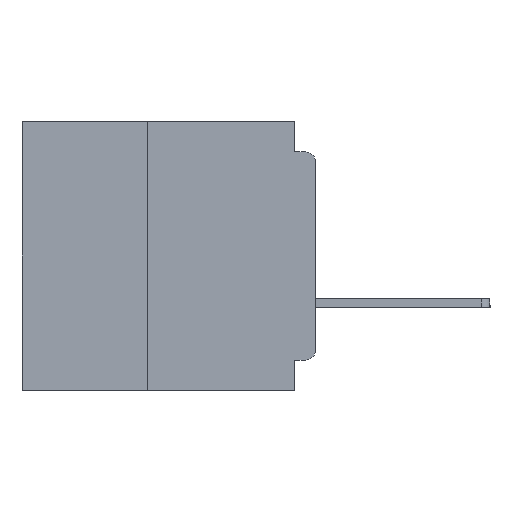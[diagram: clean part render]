
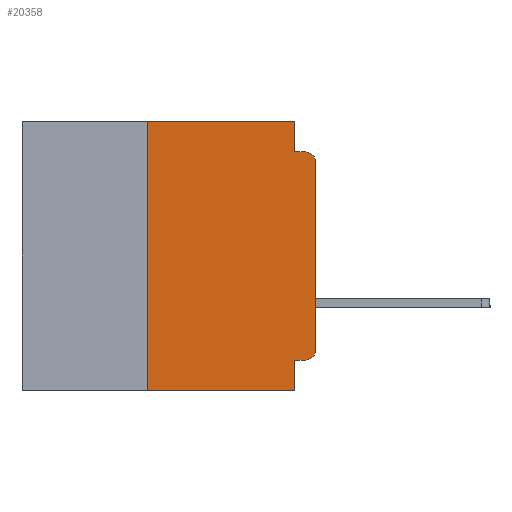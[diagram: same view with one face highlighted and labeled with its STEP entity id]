
A CAD part, left-side view. The second image highlights one B-rep face of the part: STEP entity #20358.
In plain terms, the highlighted planar face has unit normal (-1, 0, 0).
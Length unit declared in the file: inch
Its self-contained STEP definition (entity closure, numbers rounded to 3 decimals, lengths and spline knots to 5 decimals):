
#135 = EDGE_CURVE ( 'NONE', #14110, #29650, #40078, .T. ) ;
#1455 = CARTESIAN_POINT ( 'NONE',  ( 0., 0.437, -0.4 ) ) ;
#1759 = VECTOR ( 'NONE', #25606, 39.37008 ) ;
#2376 = CARTESIAN_POINT ( 'NONE',  ( 0., 0., -0.06 ) ) ;
#2440 = VERTEX_POINT ( 'NONE', #45266 ) ;
#2947 = VECTOR ( 'NONE', #39815, 39.37008 ) ;
#3290 = CARTESIAN_POINT ( 'NONE',  ( 0., 0., -0.34 ) ) ;
#3798 = ORIENTED_EDGE ( 'NONE', *, *, #34696, .F. ) ;
#3933 = VERTEX_POINT ( 'NONE', #2376 ) ;
#4945 = DIRECTION ( 'NONE',  ( 1., 0., 0. ) ) ;
#4977 = DIRECTION ( 'NONE',  ( 0., 0., 1. ) ) ;
#5087 = CARTESIAN_POINT ( 'NONE',  ( 0., 0.031, -0.4 ) ) ;
#6146 = LINE ( 'NONE', #5087, #36688 ) ;
#6580 = FACE_OUTER_BOUND ( 'NONE', #43838, .T. ) ;
#6776 = ORIENTED_EDGE ( 'NONE', *, *, #35866, .T. ) ;
#7638 = ORIENTED_EDGE ( 'NONE', *, *, #19203, .T. ) ;
#7795 = DIRECTION ( 'NONE',  ( 0., -1., 0. ) ) ;
#8506 = ORIENTED_EDGE ( 'NONE', *, *, #38034, .F. ) ;
#8842 = PLANE ( 'NONE',  #8988 ) ;
#8988 = AXIS2_PLACEMENT_3D ( 'NONE', #28904, #4945, #32868 ) ;
#9534 = DIRECTION ( 'NONE',  ( -1., 0., 0. ) ) ;
#10682 = ORIENTED_EDGE ( 'NONE', *, *, #41128, .T. ) ;
#11262 = CARTESIAN_POINT ( 'NONE',  ( 0., 0.015, -0.045 ) ) ;
#11462 = LINE ( 'NONE', #33960, #23397 ) ;
#11940 = CARTESIAN_POINT ( 'NONE',  ( 0., 0.015, -0.355 ) ) ;
#13378 = DIRECTION ( 'NONE',  ( -1., 0., 0. ) ) ;
#13646 = VERTEX_POINT ( 'NONE', #14329 ) ;
#13850 = LINE ( 'NONE', #1455, #1759 ) ;
#14110 = VERTEX_POINT ( 'NONE', #41070 ) ;
#14329 = CARTESIAN_POINT ( 'NONE',  ( 0., 0.031, -0.4 ) ) ;
#14405 = VERTEX_POINT ( 'NONE', #11262 ) ;
#15623 = LINE ( 'NONE', #32900, #24972 ) ;
#16126 = CARTESIAN_POINT ( 'NONE',  ( 0., 0., -0.045 ) ) ;
#16718 = VECTOR ( 'NONE', #7795, 39.37008 ) ;
#17193 = EDGE_CURVE ( 'NONE', #33635, #2440, #40490, .T. ) ;
#18382 = CARTESIAN_POINT ( 'NONE',  ( 0., 0.031, 0. ) ) ;
#19068 = VECTOR ( 'NONE', #36081, 39.37008 ) ;
#19203 = EDGE_CURVE ( 'NONE', #43689, #31374, #21826, .T. ) ;
#19774 = VERTEX_POINT ( 'NONE', #44609 ) ;
#20358 = ADVANCED_FACE ( 'NONE', ( #6580 ), #8842, .F. ) ;
#21826 = CIRCLE ( 'NONE', #22100, 0.015 ) ;
#22100 = AXIS2_PLACEMENT_3D ( 'NONE', #37120, #13378, #41073 ) ;
#22409 = CARTESIAN_POINT ( 'NONE',  ( 0., 0.031, -0.045 ) ) ;
#23397 = VECTOR ( 'NONE', #37930, 39.37008 ) ;
#24972 = VECTOR ( 'NONE', #4977, 39.37008 ) ;
#25606 = DIRECTION ( 'NONE',  ( 0., -1., 0. ) ) ;
#25615 = LINE ( 'NONE', #16126, #2947 ) ;
#26631 = ORIENTED_EDGE ( 'NONE', *, *, #43875, .T. ) ;
#27282 = LINE ( 'NONE', #47132, #16718 ) ;
#28904 = CARTESIAN_POINT ( 'NONE',  ( 0., 0.437, 0. ) ) ;
#29454 = CIRCLE ( 'NONE', #30776, 0.015 ) ;
#29650 = VERTEX_POINT ( 'NONE', #22409 ) ;
#30022 = VECTOR ( 'NONE', #50939, 39.37008 ) ;
#30776 = AXIS2_PLACEMENT_3D ( 'NONE', #33345, #9534, #37321 ) ;
#30788 = CARTESIAN_POINT ( 'NONE',  ( 0., 0.25, -0.4 ) ) ;
#31374 = VERTEX_POINT ( 'NONE', #3290 ) ;
#32868 = DIRECTION ( 'NONE',  ( 0., 0., -1. ) ) ;
#32897 = ORIENTED_EDGE ( 'NONE', *, *, #135, .F. ) ;
#32900 = CARTESIAN_POINT ( 'NONE',  ( 0., 0., 0. ) ) ;
#33345 = CARTESIAN_POINT ( 'NONE',  ( 0., 0.015, -0.06 ) ) ;
#33635 = VERTEX_POINT ( 'NONE', #30788 ) ;
#33960 = CARTESIAN_POINT ( 'NONE',  ( 0., 0., -0.355 ) ) ;
#34696 = EDGE_CURVE ( 'NONE', #43689, #19774, #11462, .T. ) ;
#35088 = ORIENTED_EDGE ( 'NONE', *, *, #17193, .F. ) ;
#35866 = EDGE_CURVE ( 'NONE', #33635, #13646, #13850, .T. ) ;
#36081 = DIRECTION ( 'NONE',  ( 0., 0., -1. ) ) ;
#36688 = VECTOR ( 'NONE', #36972, 39.37008 ) ;
#36899 = ORIENTED_EDGE ( 'NONE', *, *, #44475, .F. ) ;
#36972 = DIRECTION ( 'NONE',  ( 0., 0., -1. ) ) ;
#37120 = CARTESIAN_POINT ( 'NONE',  ( 0., 0.015, -0.34 ) ) ;
#37321 = DIRECTION ( 'NONE',  ( 0., 0., -1. ) ) ;
#37930 = DIRECTION ( 'NONE',  ( 0., 1., 0. ) ) ;
#38034 = EDGE_CURVE ( 'NONE', #2440, #14110, #27282, .T. ) ;
#39815 = DIRECTION ( 'NONE',  ( 0., -1., 0. ) ) ;
#40078 = LINE ( 'NONE', #18382, #19068 ) ;
#40490 = LINE ( 'NONE', #47008, #30022 ) ;
#41070 = CARTESIAN_POINT ( 'NONE',  ( 0., 0.031, 0. ) ) ;
#41073 = DIRECTION ( 'NONE',  ( 0., 0., -1. ) ) ;
#41128 = EDGE_CURVE ( 'NONE', #3933, #14405, #29454, .T. ) ;
#43689 = VERTEX_POINT ( 'NONE', #11940 ) ;
#43720 = EDGE_CURVE ( 'NONE', #29650, #14405, #25615, .T. ) ;
#43838 = EDGE_LOOP ( 'NONE', ( #26631, #10682, #49598, #32897, #8506, #35088, #6776, #36899, #3798, #7638 ) ) ;
#43875 = EDGE_CURVE ( 'NONE', #31374, #3933, #15623, .T. ) ;
#44475 = EDGE_CURVE ( 'NONE', #19774, #13646, #6146, .T. ) ;
#44609 = CARTESIAN_POINT ( 'NONE',  ( 0., 0.031, -0.355 ) ) ;
#45266 = CARTESIAN_POINT ( 'NONE',  ( 0., 0.25, 0. ) ) ;
#47008 = CARTESIAN_POINT ( 'NONE',  ( 0., 0.25, -0.4 ) ) ;
#47132 = CARTESIAN_POINT ( 'NONE',  ( 0., 0.437, 0. ) ) ;
#49598 = ORIENTED_EDGE ( 'NONE', *, *, #43720, .F. ) ;
#50939 = DIRECTION ( 'NONE',  ( 0., 0., 1. ) ) ;
